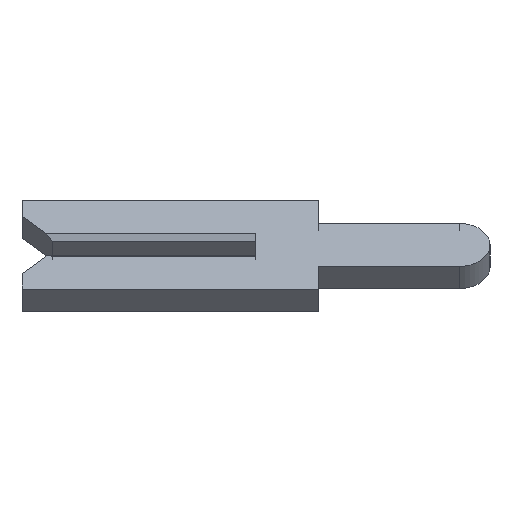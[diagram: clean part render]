
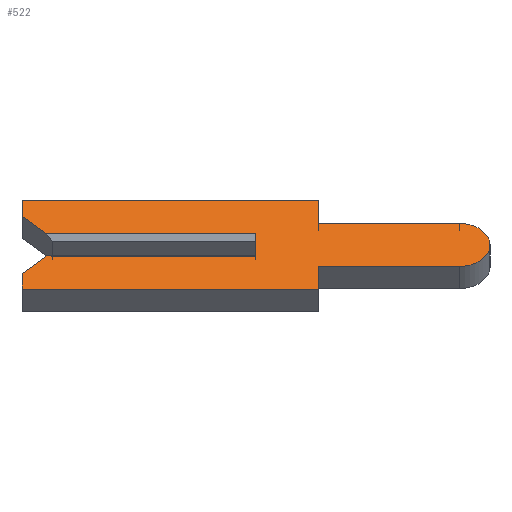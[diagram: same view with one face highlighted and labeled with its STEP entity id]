
A CAD part, left-side view. The second image highlights one B-rep face of the part: STEP entity #522.
In plain terms, the highlighted face is planar.
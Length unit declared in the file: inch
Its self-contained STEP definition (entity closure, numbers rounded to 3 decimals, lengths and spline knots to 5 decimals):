
#7 = EDGE_CURVE ( 'NONE', #1247, #792, #835, .T. ) ;
#31 = EDGE_CURVE ( 'NONE', #776, #1002, #183, .T. ) ;
#33 = LINE ( 'NONE', #1553, #621 ) ;
#51 = VERTEX_POINT ( 'NONE', #233 ) ;
#87 = VERTEX_POINT ( 'NONE', #849 ) ;
#94 = DIRECTION ( 'NONE',  ( 0., 0., 1. ) ) ;
#98 = DIRECTION ( 'NONE',  ( 0., -1., 0. ) ) ;
#100 = CARTESIAN_POINT ( 'NONE',  ( -0.01, -0.04, 0.04 ) ) ;
#111 = LINE ( 'NONE', #473, #1362 ) ;
#122 = LINE ( 'NONE', #712, #1404 ) ;
#126 = CARTESIAN_POINT ( 'NONE',  ( -0.01, -0.04, -0.04 ) ) ;
#137 = DIRECTION ( 'NONE',  ( 0., 0., 1. ) ) ;
#163 = VERTEX_POINT ( 'NONE', #126 ) ;
#167 = LINE ( 'NONE', #1450, #1264 ) ;
#179 = ORIENTED_EDGE ( 'NONE', *, *, #511, .F. ) ;
#183 = LINE ( 'NONE', #600, #1130 ) ;
#200 = CARTESIAN_POINT ( 'NONE',  ( -0.01, -0.1305, -0.01 ) ) ;
#209 = EDGE_CURVE ( 'NONE', #1275, #535, #748, .T. ) ;
#230 = CARTESIAN_POINT ( 'NONE',  ( -0.01, 0.134, 0.01 ) ) ;
#233 = CARTESIAN_POINT ( 'NONE',  ( -0.01, -0.04, -0.0195 ) ) ;
#261 = ORIENTED_EDGE ( 'NONE', *, *, #1527, .F. ) ;
#273 = EDGE_CURVE ( 'NONE', #906, #792, #540, .T. ) ;
#281 = AXIS2_PLACEMENT_3D ( 'NONE', #711, #903, #853 ) ;
#322 = CARTESIAN_POINT ( 'NONE',  ( -0.01, 0.15, -0.026 ) ) ;
#328 = CARTESIAN_POINT ( 'NONE',  ( -0.01, 0.15, 0.04 ) ) ;
#341 = CARTESIAN_POINT ( 'NONE',  ( -0.01, 0.134, -0.01 ) ) ;
#347 = ORIENTED_EDGE ( 'NONE', *, *, #875, .F. ) ;
#351 = DIRECTION ( 'NONE',  ( 0., -1., 0. ) ) ;
#372 = EDGE_CURVE ( 'NONE', #1319, #902, #111, .T. ) ;
#432 = EDGE_LOOP ( 'NONE', ( #545, #1351, #657, #510, #1000, #261, #179, #347, #1445, #1513, #1517, #624, #1529, #1071 ) ) ;
#445 = CARTESIAN_POINT ( 'NONE',  ( -0.01, 0., -0.01 ) ) ;
#473 = CARTESIAN_POINT ( 'NONE',  ( -0.01, 0.15, 0.04 ) ) ;
#475 = CARTESIAN_POINT ( 'NONE',  ( -0.01, 0.15, 0.01 ) ) ;
#482 = VECTOR ( 'NONE', #94, 39.37008 ) ;
#498 = CARTESIAN_POINT ( 'NONE',  ( -0.01, -0.1305, 0. ) ) ;
#510 = ORIENTED_EDGE ( 'NONE', *, *, #31, .F. ) ;
#511 = EDGE_CURVE ( 'NONE', #51, #163, #1117, .T. ) ;
#513 = VECTOR ( 'NONE', #687, 39.37008 ) ;
#522 = ADVANCED_FACE ( 'NONE', ( #1530 ), #603, .F. ) ;
#535 = VERTEX_POINT ( 'NONE', #1460 ) ;
#540 = LINE ( 'NONE', #1235, #639 ) ;
#545 = ORIENTED_EDGE ( 'NONE', *, *, #7, .T. ) ;
#565 = CARTESIAN_POINT ( 'NONE',  ( -0.01, -0.04, 0.04 ) ) ;
#598 = DIRECTION ( 'NONE',  ( 0., 0., 1. ) ) ;
#600 = CARTESIAN_POINT ( 'NONE',  ( -0.01, 0.1305, -0.0065 ) ) ;
#603 = PLANE ( 'NONE',  #281 ) ;
#621 = VECTOR ( 'NONE', #941, 39.37008 ) ;
#624 = ORIENTED_EDGE ( 'NONE', *, *, #372, .F. ) ;
#639 = VECTOR ( 'NONE', #137, 39.37008 ) ;
#657 = ORIENTED_EDGE ( 'NONE', *, *, #1302, .F. ) ;
#669 = LINE ( 'NONE', #565, #1484 ) ;
#687 = DIRECTION ( 'NONE',  ( 0., 0.707, 0.707 ) ) ;
#698 = CARTESIAN_POINT ( 'NONE',  ( -0.01, 0.15, -0.04 ) ) ;
#699 = CARTESIAN_POINT ( 'NONE',  ( -0.01, 0.15, -0.026 ) ) ;
#711 = CARTESIAN_POINT ( 'NONE',  ( -0.01, -0.1305, 0. ) ) ;
#712 = CARTESIAN_POINT ( 'NONE',  ( -0.01, 0.15, 0.026 ) ) ;
#714 = VECTOR ( 'NONE', #98, 39.37008 ) ;
#717 = DIRECTION ( 'NONE',  ( 0., -0.707, 0.707 ) ) ;
#738 = VERTEX_POINT ( 'NONE', #1248 ) ;
#748 = CIRCLE ( 'NONE', #1359, 0.0195 ) ;
#776 = VERTEX_POINT ( 'NONE', #322 ) ;
#792 = VERTEX_POINT ( 'NONE', #1315 ) ;
#794 = VECTOR ( 'NONE', #1055, 39.37008 ) ;
#804 = EDGE_CURVE ( 'NONE', #738, #1275, #167, .T. ) ;
#835 = LINE ( 'NONE', #475, #1449 ) ;
#849 = CARTESIAN_POINT ( 'NONE',  ( -0.01, 0.15, 0.026 ) ) ;
#853 = DIRECTION ( 'NONE',  ( 0., 0., -1. ) ) ;
#875 = EDGE_CURVE ( 'NONE', #535, #51, #1382, .T. ) ;
#902 = VERTEX_POINT ( 'NONE', #100 ) ;
#903 = DIRECTION ( 'NONE',  ( 1., 0., 0. ) ) ;
#906 = VERTEX_POINT ( 'NONE', #445 ) ;
#923 = EDGE_CURVE ( 'NONE', #1436, #776, #1221, .T. ) ;
#934 = DIRECTION ( 'NONE',  ( 0., 0., -1. ) ) ;
#941 = DIRECTION ( 'NONE',  ( 0., 1., 0. ) ) ;
#963 = EDGE_CURVE ( 'NONE', #1247, #87, #1493, .T. ) ;
#989 = DIRECTION ( 'NONE',  ( 1., 0., 0. ) ) ;
#1000 = ORIENTED_EDGE ( 'NONE', *, *, #923, .F. ) ;
#1002 = VERTEX_POINT ( 'NONE', #341 ) ;
#1055 = DIRECTION ( 'NONE',  ( 0., 1., 0. ) ) ;
#1071 = ORIENTED_EDGE ( 'NONE', *, *, #963, .F. ) ;
#1082 = DIRECTION ( 'NONE',  ( 0., -1., 0. ) ) ;
#1087 = CARTESIAN_POINT ( 'NONE',  ( -0.01, -0.04, -0.0195 ) ) ;
#1117 = LINE ( 'NONE', #1219, #1167 ) ;
#1126 = LINE ( 'NONE', #200, #714 ) ;
#1128 = CARTESIAN_POINT ( 'NONE',  ( -0.01, -0.1305, 0.0195 ) ) ;
#1130 = VECTOR ( 'NONE', #717, 39.37008 ) ;
#1142 = EDGE_CURVE ( 'NONE', #87, #1319, #122, .T. ) ;
#1167 = VECTOR ( 'NONE', #1566, 39.37008 ) ;
#1219 = CARTESIAN_POINT ( 'NONE',  ( -0.01, -0.04, -0.04 ) ) ;
#1221 = LINE ( 'NONE', #699, #482 ) ;
#1235 = CARTESIAN_POINT ( 'NONE',  ( -0.01, 0., 0.0065 ) ) ;
#1247 = VERTEX_POINT ( 'NONE', #230 ) ;
#1248 = CARTESIAN_POINT ( 'NONE',  ( -0.01, -0.04, 0.0195 ) ) ;
#1264 = VECTOR ( 'NONE', #351, 39.37008 ) ;
#1275 = VERTEX_POINT ( 'NONE', #1128 ) ;
#1302 = EDGE_CURVE ( 'NONE', #1002, #906, #1126, .T. ) ;
#1307 = CARTESIAN_POINT ( 'NONE',  ( -0.01, 0.1305, 0.0065 ) ) ;
#1315 = CARTESIAN_POINT ( 'NONE',  ( -0.01, 0., 0.01 ) ) ;
#1319 = VERTEX_POINT ( 'NONE', #328 ) ;
#1330 = DIRECTION ( 'NONE',  ( 0., -1., 0. ) ) ;
#1351 = ORIENTED_EDGE ( 'NONE', *, *, #273, .F. ) ;
#1359 = AXIS2_PLACEMENT_3D ( 'NONE', #498, #989, #1481 ) ;
#1362 = VECTOR ( 'NONE', #1082, 39.37008 ) ;
#1382 = LINE ( 'NONE', #1087, #794 ) ;
#1404 = VECTOR ( 'NONE', #598, 39.37008 ) ;
#1436 = VERTEX_POINT ( 'NONE', #698 ) ;
#1445 = ORIENTED_EDGE ( 'NONE', *, *, #209, .F. ) ;
#1449 = VECTOR ( 'NONE', #1330, 39.37008 ) ;
#1450 = CARTESIAN_POINT ( 'NONE',  ( -0.01, -0.04, 0.0195 ) ) ;
#1460 = CARTESIAN_POINT ( 'NONE',  ( -0.01, -0.1305, -0.0195 ) ) ;
#1481 = DIRECTION ( 'NONE',  ( 0., 0., -1. ) ) ;
#1484 = VECTOR ( 'NONE', #934, 39.37008 ) ;
#1493 = LINE ( 'NONE', #1307, #513 ) ;
#1498 = EDGE_CURVE ( 'NONE', #902, #738, #669, .T. ) ;
#1513 = ORIENTED_EDGE ( 'NONE', *, *, #804, .F. ) ;
#1517 = ORIENTED_EDGE ( 'NONE', *, *, #1498, .F. ) ;
#1527 = EDGE_CURVE ( 'NONE', #163, #1436, #33, .T. ) ;
#1529 = ORIENTED_EDGE ( 'NONE', *, *, #1142, .F. ) ;
#1530 = FACE_OUTER_BOUND ( 'NONE', #432, .T. ) ;
#1553 = CARTESIAN_POINT ( 'NONE',  ( -0.01, 0.15, -0.04 ) ) ;
#1566 = DIRECTION ( 'NONE',  ( 0., 0., -1. ) ) ;
